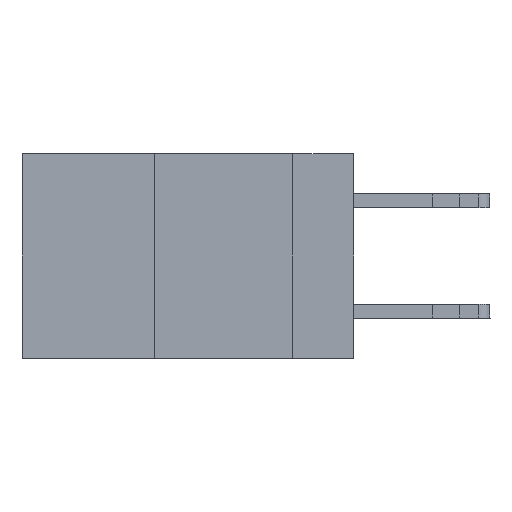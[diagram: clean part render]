
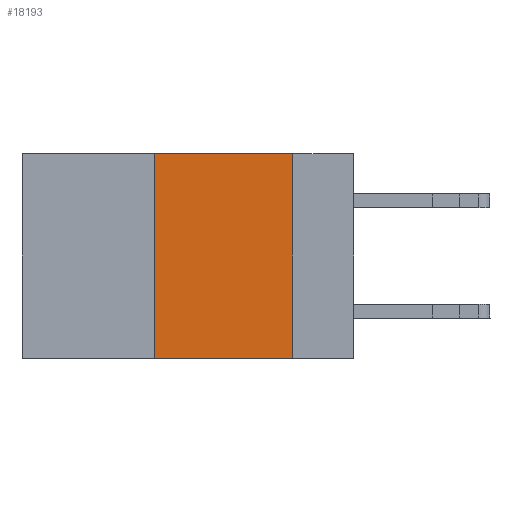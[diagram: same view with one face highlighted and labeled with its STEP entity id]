
A CAD part, left-side view. The second image highlights one B-rep face of the part: STEP entity #18193.
In plain terms, the highlighted planar face has unit normal (-1, 0, 0).
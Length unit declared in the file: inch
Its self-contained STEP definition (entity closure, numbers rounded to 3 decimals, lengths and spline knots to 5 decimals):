
#5 = VECTOR ( 'NONE', #10861, 39.37008 ) ;
#1108 = EDGE_CURVE ( 'NONE', #4911, #6120, #3620, .T. ) ;
#3620 = LINE ( 'NONE', #20389, #7398 ) ;
#4118 = DIRECTION ( 'NONE',  ( 1., 0., 0. ) ) ;
#4200 = CARTESIAN_POINT ( 'NONE',  ( 0., 0.11, 0. ) ) ;
#4895 = CARTESIAN_POINT ( 'NONE',  ( 0., 0.36, -0.37 ) ) ;
#4911 = VERTEX_POINT ( 'NONE', #4200 ) ;
#5292 = EDGE_LOOP ( 'NONE', ( #8354, #8821, #9014, #9398 ) ) ;
#5837 = LINE ( 'NONE', #16685, #19891 ) ;
#6090 = LINE ( 'NONE', #14583, #5 ) ;
#6120 = VERTEX_POINT ( 'NONE', #10540 ) ;
#7398 = VECTOR ( 'NONE', #23260, 39.37008 ) ;
#8341 = VERTEX_POINT ( 'NONE', #21109 ) ;
#8354 = ORIENTED_EDGE ( 'NONE', *, *, #1108, .F. ) ;
#8821 = ORIENTED_EDGE ( 'NONE', *, *, #21768, .F. ) ;
#9014 = ORIENTED_EDGE ( 'NONE', *, *, #9796, .F. ) ;
#9398 = ORIENTED_EDGE ( 'NONE', *, *, #13564, .T. ) ;
#9796 = EDGE_CURVE ( 'NONE', #10342, #8341, #6090, .T. ) ;
#10342 = VERTEX_POINT ( 'NONE', #4895 ) ;
#10540 = CARTESIAN_POINT ( 'NONE',  ( 0., 0.11, -0.37 ) ) ;
#10861 = DIRECTION ( 'NONE',  ( 0., 0., 1. ) ) ;
#11509 = CARTESIAN_POINT ( 'NONE',  ( 0., 0.6, 0. ) ) ;
#12237 = AXIS2_PLACEMENT_3D ( 'NONE', #11509, #4118, #17023 ) ;
#13564 = EDGE_CURVE ( 'NONE', #10342, #6120, #21663, .T. ) ;
#14583 = CARTESIAN_POINT ( 'NONE',  ( 0., 0.36, 0. ) ) ;
#15228 = PLANE ( 'NONE',  #12237 ) ;
#15238 = FACE_OUTER_BOUND ( 'NONE', #5292, .T. ) ;
#16685 = CARTESIAN_POINT ( 'NONE',  ( 0., 0.6, 0. ) ) ;
#17023 = DIRECTION ( 'NONE',  ( 0., 0., -1. ) ) ;
#17807 = CARTESIAN_POINT ( 'NONE',  ( 0., 0.6, -0.37 ) ) ;
#18193 = ADVANCED_FACE ( 'NONE', ( #15238 ), #15228, .F. ) ;
#18367 = DIRECTION ( 'NONE',  ( 0., -1., 0. ) ) ;
#19891 = VECTOR ( 'NONE', #18367, 39.37008 ) ;
#20389 = CARTESIAN_POINT ( 'NONE',  ( 0., 0.11, 0. ) ) ;
#21103 = VECTOR ( 'NONE', #21469, 39.37008 ) ;
#21109 = CARTESIAN_POINT ( 'NONE',  ( 0., 0.36, 0. ) ) ;
#21469 = DIRECTION ( 'NONE',  ( 0., -1., 0. ) ) ;
#21663 = LINE ( 'NONE', #17807, #21103 ) ;
#21768 = EDGE_CURVE ( 'NONE', #8341, #4911, #5837, .T. ) ;
#23260 = DIRECTION ( 'NONE',  ( 0., 0., -1. ) ) ;
